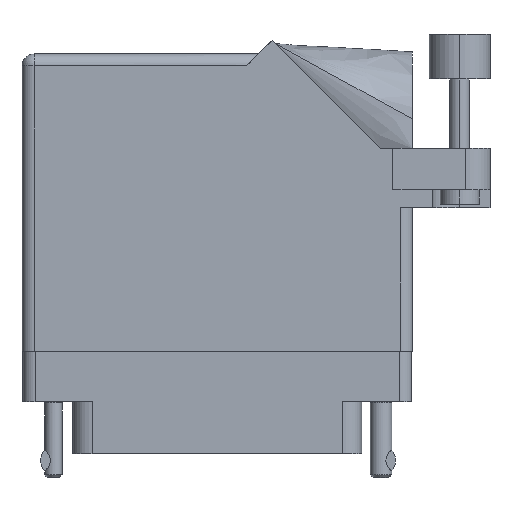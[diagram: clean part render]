
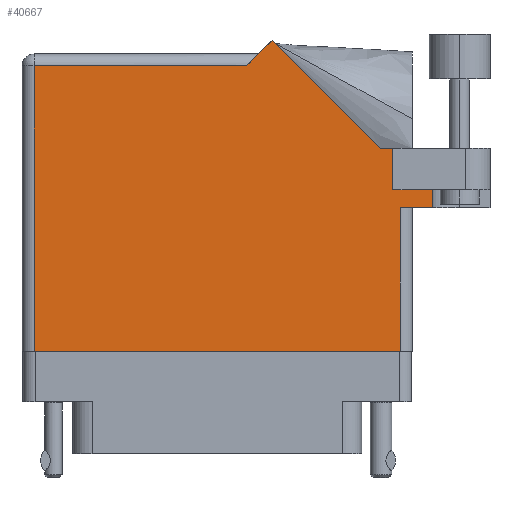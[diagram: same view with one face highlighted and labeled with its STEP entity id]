
A CAD part, front view. The second image highlights one B-rep face of the part: STEP entity #40667.
In plain terms, the highlighted face is planar.
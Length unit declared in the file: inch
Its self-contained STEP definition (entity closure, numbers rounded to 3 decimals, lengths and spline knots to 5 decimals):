
#784 = CARTESIAN_POINT ( 'NONE',  ( 2.1115, 0.737, 0. ) ) ;
#1323 = LINE ( 'NONE', #38844, #39089 ) ;
#1400 = DIRECTION ( 'NONE',  ( 0., 1., 0. ) ) ;
#1454 = DIRECTION ( 'NONE',  ( 0., 0., -1. ) ) ;
#3135 = LINE ( 'NONE', #18980, #14968 ) ;
#3319 = ORIENTED_EDGE ( 'NONE', *, *, #39229, .T. ) ;
#3821 = DIRECTION ( 'NONE',  ( 1., 0., 0. ) ) ;
#4055 = VECTOR ( 'NONE', #26918, 39.37008 ) ;
#4745 = DIRECTION ( 'NONE',  ( -1., 0., 0. ) ) ;
#4901 = DIRECTION ( 'NONE',  ( -1., 0., 0. ) ) ;
#5150 = VECTOR ( 'NONE', #18438, 39.37008 ) ;
#5159 = EDGE_CURVE ( 'NONE', #15039, #17162, #41594, .T. ) ;
#5340 = VERTEX_POINT ( 'NONE', #29782 ) ;
#5487 = EDGE_CURVE ( 'NONE', #15912, #12134, #18381, .T. ) ;
#6443 = CARTESIAN_POINT ( 'NONE',  ( 2.1115, 0.831, 0. ) ) ;
#8004 = CARTESIAN_POINT ( 'NONE',  ( 1.91, 0.831, 0. ) ) ;
#8325 = DIRECTION ( 'NONE',  ( -0.707, -0.707, 0. ) ) ;
#9434 = VECTOR ( 'NONE', #1400, 39.37008 ) ;
#9520 = CARTESIAN_POINT ( 'NONE',  ( 0., 0., 0. ) ) ;
#9824 = VERTEX_POINT ( 'NONE', #26855 ) ;
#11493 = LINE ( 'NONE', #31867, #26124 ) ;
#11583 = CARTESIAN_POINT ( 'NONE',  ( 0.062, 0., 0. ) ) ;
#12134 = VERTEX_POINT ( 'NONE', #36420 ) ;
#12437 = VERTEX_POINT ( 'NONE', #6443 ) ;
#12997 = DIRECTION ( 'NONE',  ( 1., 0., 0. ) ) ;
#13888 = VERTEX_POINT ( 'NONE', #24152 ) ;
#14252 = EDGE_CURVE ( 'NONE', #12134, #19457, #3135, .T. ) ;
#14968 = VECTOR ( 'NONE', #25935, 39.37008 ) ;
#15010 = FACE_OUTER_BOUND ( 'NONE', #28019, .T. ) ;
#15039 = VERTEX_POINT ( 'NONE', #16819 ) ;
#15912 = VERTEX_POINT ( 'NONE', #37010 ) ;
#16211 = LINE ( 'NONE', #41801, #36736 ) ;
#16318 = EDGE_CURVE ( 'NONE', #13888, #12437, #22982, .T. ) ;
#16609 = VERTEX_POINT ( 'NONE', #37550 ) ;
#16800 = CARTESIAN_POINT ( 'NONE',  ( 1.84442, 1.044, 0. ) ) ;
#16819 = CARTESIAN_POINT ( 'NONE',  ( 1.91, 1.044, 0. ) ) ;
#16905 = EDGE_CURVE ( 'NONE', #9824, #5340, #1323, .T. ) ;
#17162 = VERTEX_POINT ( 'NONE', #34160 ) ;
#18082 = LINE ( 'NONE', #16800, #4055 ) ;
#18381 = LINE ( 'NONE', #30667, #39962 ) ;
#18438 = DIRECTION ( 'NONE',  ( 1., 0., 0. ) ) ;
#18980 = CARTESIAN_POINT ( 'NONE',  ( 0.062, 0., 0. ) ) ;
#19256 = VERTEX_POINT ( 'NONE', #784 ) ;
#19457 = VERTEX_POINT ( 'NONE', #11583 ) ;
#20047 = ORIENTED_EDGE ( 'NONE', *, *, #16318, .F. ) ;
#21648 = DIRECTION ( 'NONE',  ( 0., 1., 0. ) ) ;
#22229 = CARTESIAN_POINT ( 'NONE',  ( 2.41, 1.044, 0. ) ) ;
#22710 = ORIENTED_EDGE ( 'NONE', *, *, #16905, .T. ) ;
#22982 = LINE ( 'NONE', #8004, #5150 ) ;
#23252 = VECTOR ( 'NONE', #4745, 39.37008 ) ;
#23476 = LINE ( 'NONE', #9520, #32093 ) ;
#23884 = EDGE_CURVE ( 'NONE', #16609, #15912, #11493, .T. ) ;
#24152 = CARTESIAN_POINT ( 'NONE',  ( 1.91, 0.831, 0. ) ) ;
#25578 = CARTESIAN_POINT ( 'NONE',  ( 0., 1.53, 0. ) ) ;
#25675 = CARTESIAN_POINT ( 'NONE',  ( 1.91, 0.831, 0. ) ) ;
#25935 = DIRECTION ( 'NONE',  ( 0., -1., 0. ) ) ;
#26124 = VECTOR ( 'NONE', #8325, 39.37008 ) ;
#26471 = CARTESIAN_POINT ( 'NONE',  ( 2.1115, 1.16177, 0. ) ) ;
#26855 = CARTESIAN_POINT ( 'NONE',  ( 1.948, 0., 0. ) ) ;
#26918 = DIRECTION ( 'NONE',  ( -0.707, 0.707, 0. ) ) ;
#28019 = EDGE_LOOP ( 'NONE', ( #28128, #22710, #3319, #39625, #20047, #37041, #30931, #32383, #42957, #33497, #44079 ) ) ;
#28128 = ORIENTED_EDGE ( 'NONE', *, *, #35609, .T. ) ;
#29782 = CARTESIAN_POINT ( 'NONE',  ( 1.948, 0.737, 0. ) ) ;
#30237 = DIRECTION ( 'NONE',  ( 0., -1., 0. ) ) ;
#30667 = CARTESIAN_POINT ( 'NONE',  ( 0., 1.468, 0. ) ) ;
#30931 = ORIENTED_EDGE ( 'NONE', *, *, #5159, .T. ) ;
#31599 = EDGE_CURVE ( 'NONE', #12437, #19256, #37580, .T. ) ;
#31867 = CARTESIAN_POINT ( 'NONE',  ( 1.217, 1.53, 0. ) ) ;
#32093 = VECTOR ( 'NONE', #12997, 39.37008 ) ;
#32151 = AXIS2_PLACEMENT_3D ( 'NONE', #25578, #1454, #4901 ) ;
#32383 = ORIENTED_EDGE ( 'NONE', *, *, #43906, .T. ) ;
#33497 = ORIENTED_EDGE ( 'NONE', *, *, #5487, .T. ) ;
#34138 = DIRECTION ( 'NONE',  ( -1., 0., 0. ) ) ;
#34160 = CARTESIAN_POINT ( 'NONE',  ( 1.84442, 1.044, 0. ) ) ;
#35609 = EDGE_CURVE ( 'NONE', #19457, #9824, #23476, .T. ) ;
#36420 = CARTESIAN_POINT ( 'NONE',  ( 0.062, 1.468, 0. ) ) ;
#36736 = VECTOR ( 'NONE', #3821, 39.37008 ) ;
#37010 = CARTESIAN_POINT ( 'NONE',  ( 1.155, 1.468, 0. ) ) ;
#37041 = ORIENTED_EDGE ( 'NONE', *, *, #44375, .T. ) ;
#37550 = CARTESIAN_POINT ( 'NONE',  ( 1.28771, 1.60071, 0. ) ) ;
#37580 = LINE ( 'NONE', #26471, #39195 ) ;
#38844 = CARTESIAN_POINT ( 'NONE',  ( 1.948, 0.737, 0. ) ) ;
#39089 = VECTOR ( 'NONE', #21648, 39.37008 ) ;
#39195 = VECTOR ( 'NONE', #30237, 39.37008 ) ;
#39229 = EDGE_CURVE ( 'NONE', #5340, #19256, #16211, .T. ) ;
#39625 = ORIENTED_EDGE ( 'NONE', *, *, #31599, .F. ) ;
#39962 = VECTOR ( 'NONE', #34138, 39.37008 ) ;
#40667 = ADVANCED_FACE ( 'NONE', ( #15010 ), #42756, .F. ) ;
#41594 = LINE ( 'NONE', #22229, #23252 ) ;
#41801 = CARTESIAN_POINT ( 'NONE',  ( 2.01, 0.737, 0. ) ) ;
#42756 = PLANE ( 'NONE',  #32151 ) ;
#42957 = ORIENTED_EDGE ( 'NONE', *, *, #23884, .T. ) ;
#43464 = LINE ( 'NONE', #25675, #9434 ) ;
#43906 = EDGE_CURVE ( 'NONE', #17162, #16609, #18082, .T. ) ;
#44079 = ORIENTED_EDGE ( 'NONE', *, *, #14252, .T. ) ;
#44375 = EDGE_CURVE ( 'NONE', #13888, #15039, #43464, .T. ) ;
